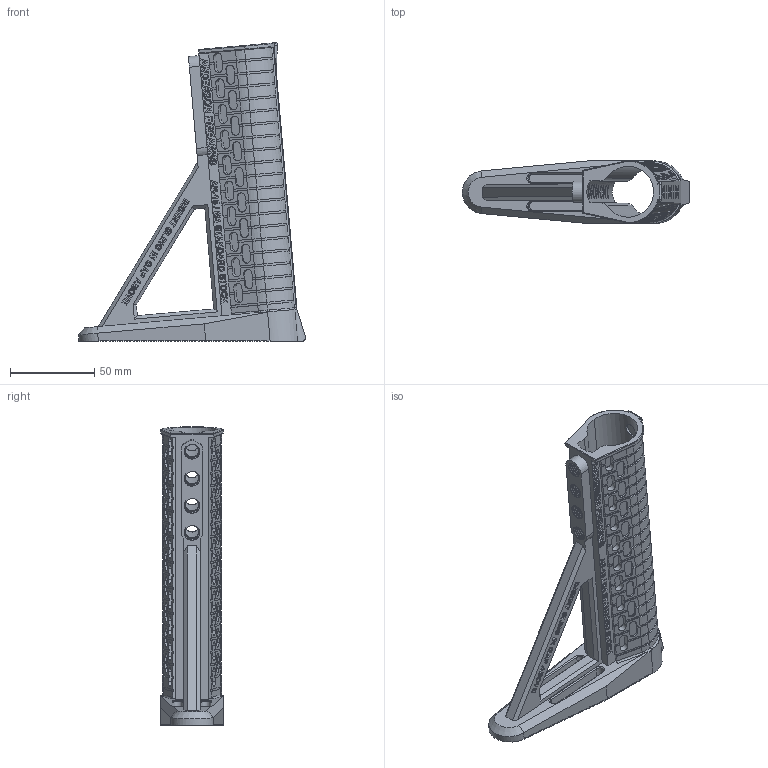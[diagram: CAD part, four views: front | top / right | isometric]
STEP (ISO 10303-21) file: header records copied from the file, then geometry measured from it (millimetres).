
FILE_DESCRIPTION (( 'STEP AP203' ), '1' );
FILE_NAME ('AF-WF-SS-PRT-001-STEP.STEP', '2020-07-22T00:05:57', ( '' ), ( '' ), 'SwSTEP 2.0', 'SolidWorks 2018', '' );
FILE_SCHEMA (( 'CONFIG_CONTROL_DESIGN' ));
Products named in the file (1): AF-WF-SS-PRT-001-STEP
Bounding box: 134.85 x 37.28 x 177.21 mm (x, y, z)
Volume: 111501 mm3; surface area: 68337.9 mm2
Topology: 1 solids, 1 shells, 2552 faces, 7045 edges, 4654 vertices
Faces by surface type: plane 1590, bspline 496, cylinder 451, torus 10, cone 5
Entity records: 115659 total; most frequent: CARTESIAN_POINT 54434, ORIENTED_EDGE 14086, DIRECTION 10350, EDGE_CURVE 7043, VECTOR 5074, LINE 5074, VERTEX_POINT 4654, EDGE_LOOP 2741
